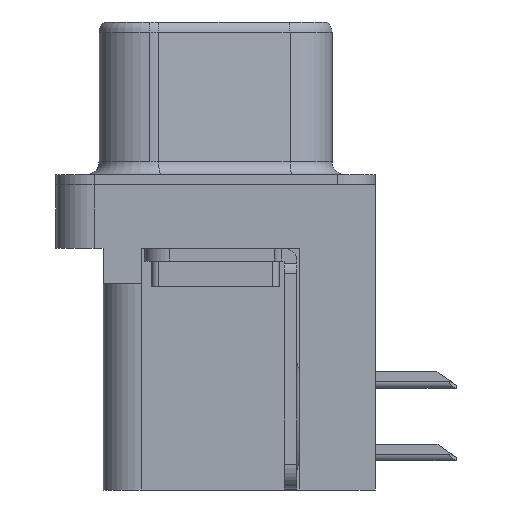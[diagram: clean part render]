
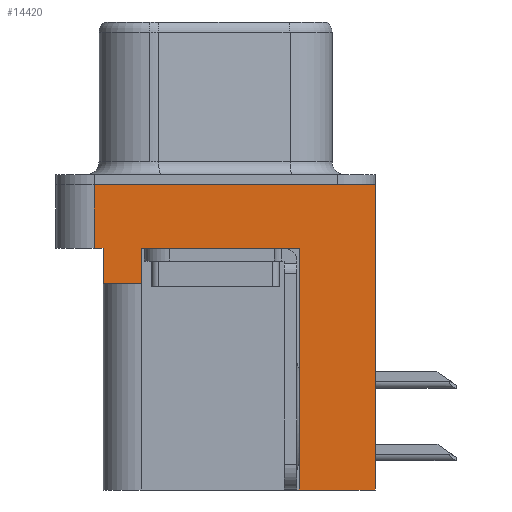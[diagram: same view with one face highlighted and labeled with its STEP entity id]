
A CAD part, left-side view. The second image highlights one B-rep face of the part: STEP entity #14420.
In plain terms, the highlighted planar face has unit normal (-1, 0, 0).
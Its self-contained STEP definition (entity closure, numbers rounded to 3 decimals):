
#186 = ORIENTED_EDGE ( 'NONE', *, *, #8594, .T. ) ;
#239 = CARTESIAN_POINT ( 'NONE',  ( -2.935, 4.775, -2.5 ) ) ;
#374 = EDGE_CURVE ( 'NONE', #15261, #19271, #12529, .T. ) ;
#407 = CARTESIAN_POINT ( 'NONE',  ( -2.935, -3.295, -12. ) ) ;
#758 = DIRECTION ( 'NONE',  ( 0., 0., 1. ) ) ;
#979 = DIRECTION ( 'NONE',  ( 0., 0., 1. ) ) ;
#1766 = LINE ( 'NONE', #14647, #18331 ) ;
#1974 = LINE ( 'NONE', #3959, #2491 ) ;
#2051 = VECTOR ( 'NONE', #2788, 1000. ) ;
#2491 = VECTOR ( 'NONE', #8982, 1000. ) ;
#2788 = DIRECTION ( 'NONE',  ( 0., 0., 1. ) ) ;
#3234 = CARTESIAN_POINT ( 'NONE',  ( -2.935, -6.275, 0. ) ) ;
#3371 = LINE ( 'NONE', #19756, #6339 ) ;
#3959 = CARTESIAN_POINT ( 'NONE',  ( -2.935, -6.275, -2.5 ) ) ;
#3974 = CARTESIAN_POINT ( 'NONE',  ( -2.935, 2.895, -2.5 ) ) ;
#4803 = DIRECTION ( 'NONE',  ( 0., -1., 0. ) ) ;
#4857 = DIRECTION ( 'NONE',  ( 0., 0., 1. ) ) ;
#5507 = VECTOR ( 'NONE', #15827, 1000. ) ;
#6001 = CARTESIAN_POINT ( 'NONE',  ( -2.935, -3.295, -12. ) ) ;
#6339 = VECTOR ( 'NONE', #4803, 1000. ) ;
#6426 = CARTESIAN_POINT ( 'NONE',  ( -2.935, 4.425, -3.9 ) ) ;
#6627 = ORIENTED_EDGE ( 'NONE', *, *, #11956, .T. ) ;
#6890 = FACE_OUTER_BOUND ( 'NONE', #8383, .T. ) ;
#6903 = EDGE_CURVE ( 'NONE', #9831, #12043, #7011, .T. ) ;
#7011 = LINE ( 'NONE', #19747, #19343 ) ;
#7068 = EDGE_CURVE ( 'NONE', #10884, #19498, #16815, .T. ) ;
#7519 = LINE ( 'NONE', #407, #20118 ) ;
#7806 = AXIS2_PLACEMENT_3D ( 'NONE', #10635, #17091, #979 ) ;
#7815 = ORIENTED_EDGE ( 'NONE', *, *, #374, .F. ) ;
#8231 = ORIENTED_EDGE ( 'NONE', *, *, #18879, .F. ) ;
#8383 = EDGE_LOOP ( 'NONE', ( #14111, #19280, #6627, #13755, #8231, #19717, #186, #7815, #15450, #19621 ) ) ;
#8594 = EDGE_CURVE ( 'NONE', #12075, #19271, #3371, .T. ) ;
#8982 = DIRECTION ( 'NONE',  ( 0., -1., 0. ) ) ;
#9831 = VERTEX_POINT ( 'NONE', #14017 ) ;
#9884 = VECTOR ( 'NONE', #17471, 1000. ) ;
#10493 = CARTESIAN_POINT ( 'NONE',  ( -2.935, 4.425, -3.9 ) ) ;
#10562 = PLANE ( 'NONE',  #7806 ) ;
#10635 = CARTESIAN_POINT ( 'NONE',  ( -2.935, -6.275, -2.5 ) ) ;
#10771 = CARTESIAN_POINT ( 'NONE',  ( -2.935, 4.425, -3.9 ) ) ;
#10822 = LINE ( 'NONE', #14041, #2051 ) ;
#10884 = VERTEX_POINT ( 'NONE', #6426 ) ;
#10956 = EDGE_CURVE ( 'NONE', #13015, #9831, #1766, .T. ) ;
#10984 = EDGE_CURVE ( 'NONE', #19061, #15261, #7519, .T. ) ;
#11196 = DIRECTION ( 'NONE',  ( 0., 0., 1. ) ) ;
#11956 = EDGE_CURVE ( 'NONE', #13015, #19498, #1974, .T. ) ;
#12043 = VERTEX_POINT ( 'NONE', #3234 ) ;
#12075 = VERTEX_POINT ( 'NONE', #3974 ) ;
#12529 = LINE ( 'NONE', #14476, #15809 ) ;
#12662 = CARTESIAN_POINT ( 'NONE',  ( -2.935, -3.295, -2.5 ) ) ;
#13015 = VERTEX_POINT ( 'NONE', #239 ) ;
#13755 = ORIENTED_EDGE ( 'NONE', *, *, #7068, .F. ) ;
#14017 = CARTESIAN_POINT ( 'NONE',  ( -2.935, 4.775, 0. ) ) ;
#14041 = CARTESIAN_POINT ( 'NONE',  ( -2.935, -6.275, -2.5 ) ) ;
#14111 = ORIENTED_EDGE ( 'NONE', *, *, #6903, .F. ) ;
#14164 = LINE ( 'NONE', #20763, #9884 ) ;
#14420 = ADVANCED_FACE ( 'NONE', ( #6890 ), #10562, .T. ) ;
#14476 = CARTESIAN_POINT ( 'NONE',  ( -2.935, -3.295, -12. ) ) ;
#14647 = CARTESIAN_POINT ( 'NONE',  ( -2.935, 4.775, -2.5 ) ) ;
#15139 = EDGE_CURVE ( 'NONE', #20365, #12075, #14164, .T. ) ;
#15261 = VERTEX_POINT ( 'NONE', #6001 ) ;
#15450 = ORIENTED_EDGE ( 'NONE', *, *, #10984, .F. ) ;
#15809 = VECTOR ( 'NONE', #4857, 1000. ) ;
#15827 = DIRECTION ( 'NONE',  ( 0., 1., 0. ) ) ;
#16559 = LINE ( 'NONE', #10771, #5507 ) ;
#16815 = LINE ( 'NONE', #10493, #17542 ) ;
#17091 = DIRECTION ( 'NONE',  ( -1., 0., 0. ) ) ;
#17471 = DIRECTION ( 'NONE',  ( 0., 0., 1. ) ) ;
#17542 = VECTOR ( 'NONE', #758, 1000. ) ;
#17934 = EDGE_CURVE ( 'NONE', #19061, #12043, #10822, .T. ) ;
#17955 = DIRECTION ( 'NONE',  ( 0., -1., 0. ) ) ;
#18331 = VECTOR ( 'NONE', #11196, 1000. ) ;
#18816 = CARTESIAN_POINT ( 'NONE',  ( -2.935, -6.275, -12. ) ) ;
#18879 = EDGE_CURVE ( 'NONE', #20365, #10884, #16559, .T. ) ;
#19061 = VERTEX_POINT ( 'NONE', #18816 ) ;
#19271 = VERTEX_POINT ( 'NONE', #12662 ) ;
#19280 = ORIENTED_EDGE ( 'NONE', *, *, #10956, .F. ) ;
#19343 = VECTOR ( 'NONE', #17955, 1000. ) ;
#19498 = VERTEX_POINT ( 'NONE', #19734 ) ;
#19621 = ORIENTED_EDGE ( 'NONE', *, *, #17934, .T. ) ;
#19717 = ORIENTED_EDGE ( 'NONE', *, *, #15139, .T. ) ;
#19734 = CARTESIAN_POINT ( 'NONE',  ( -2.935, 4.425, -2.5 ) ) ;
#19747 = CARTESIAN_POINT ( 'NONE',  ( -2.935, -6.275, 0. ) ) ;
#19756 = CARTESIAN_POINT ( 'NONE',  ( -2.935, -6.275, -2.5 ) ) ;
#19803 = DIRECTION ( 'NONE',  ( 0., 1., 0. ) ) ;
#20055 = CARTESIAN_POINT ( 'NONE',  ( -2.935, 2.895, -3.9 ) ) ;
#20118 = VECTOR ( 'NONE', #19803, 1000. ) ;
#20365 = VERTEX_POINT ( 'NONE', #20055 ) ;
#20763 = CARTESIAN_POINT ( 'NONE',  ( -2.935, 2.895, -3.9 ) ) ;
